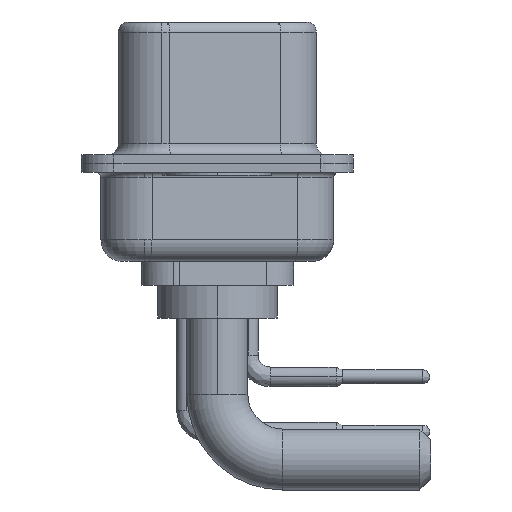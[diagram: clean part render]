
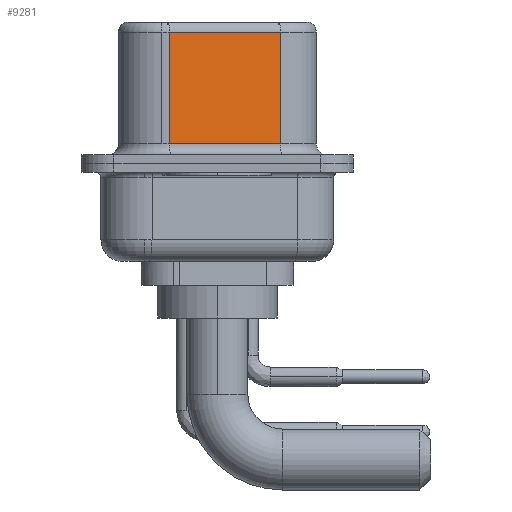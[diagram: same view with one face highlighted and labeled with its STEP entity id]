
A CAD part, left-side view. The second image highlights one B-rep face of the part: STEP entity #9281.
In plain terms, the highlighted planar face has unit normal (-0.985, -0.174, 0).
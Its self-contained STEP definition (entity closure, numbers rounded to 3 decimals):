
#72 = VERTEX_POINT ( 'NONE', #8253 ) ;
#174 = EDGE_LOOP ( 'NONE', ( #11811, #11047, #14633, #18076 ) ) ;
#455 = VECTOR ( 'NONE', #17280, 1000. ) ;
#1044 = AXIS2_PLACEMENT_3D ( 'NONE', #17611, #1335, #7945 ) ;
#1335 = DIRECTION ( 'NONE',  ( 0.985, 0.174, 0. ) ) ;
#3132 = CARTESIAN_POINT ( 'NONE',  ( 4.58, -2.897, 6.02 ) ) ;
#3667 = EDGE_CURVE ( 'NONE', #16047, #14446, #4956, .T. ) ;
#4437 = CARTESIAN_POINT ( 'NONE',  ( 3.68, 2.203, 6.52 ) ) ;
#4581 = CARTESIAN_POINT ( 'NONE',  ( 4.58, -2.897, 6.52 ) ) ;
#4956 = LINE ( 'NONE', #9182, #6905 ) ;
#6149 = DIRECTION ( 'NONE',  ( 0., 0., -1. ) ) ;
#6905 = VECTOR ( 'NONE', #19097, 1000. ) ;
#7233 = EDGE_CURVE ( 'NONE', #72, #16047, #22305, .T. ) ;
#7945 = DIRECTION ( 'NONE',  ( -0.174, 0.985, 0. ) ) ;
#8253 = CARTESIAN_POINT ( 'NONE',  ( 3.68, 2.203, 6.02 ) ) ;
#8675 = CARTESIAN_POINT ( 'NONE',  ( 3.68, 2.203, 0.9 ) ) ;
#9182 = CARTESIAN_POINT ( 'NONE',  ( 4.58, -2.897, 0.9 ) ) ;
#9209 = CARTESIAN_POINT ( 'NONE',  ( 4.58, -2.897, 6.02 ) ) ;
#9281 = ADVANCED_FACE ( 'NONE', ( #13507 ), #22103, .F. ) ;
#10082 = EDGE_CURVE ( 'NONE', #17493, #14446, #25188, .T. ) ;
#11047 = ORIENTED_EDGE ( 'NONE', *, *, #17376, .T. ) ;
#11589 = LINE ( 'NONE', #9209, #455 ) ;
#11811 = ORIENTED_EDGE ( 'NONE', *, *, #10082, .F. ) ;
#12910 = DIRECTION ( 'NONE',  ( 0., 0., -1. ) ) ;
#13507 = FACE_OUTER_BOUND ( 'NONE', #174, .T. ) ;
#14446 = VERTEX_POINT ( 'NONE', #17916 ) ;
#14459 = VECTOR ( 'NONE', #6149, 1000. ) ;
#14633 = ORIENTED_EDGE ( 'NONE', *, *, #7233, .T. ) ;
#16047 = VERTEX_POINT ( 'NONE', #8675 ) ;
#17280 = DIRECTION ( 'NONE',  ( -0.174, 0.985, 0. ) ) ;
#17376 = EDGE_CURVE ( 'NONE', #17493, #72, #11589, .T. ) ;
#17493 = VERTEX_POINT ( 'NONE', #3132 ) ;
#17611 = CARTESIAN_POINT ( 'NONE',  ( 4.58, -2.897, 6.52 ) ) ;
#17916 = CARTESIAN_POINT ( 'NONE',  ( 4.58, -2.897, 0.9 ) ) ;
#18076 = ORIENTED_EDGE ( 'NONE', *, *, #3667, .T. ) ;
#19097 = DIRECTION ( 'NONE',  ( 0.174, -0.985, 0. ) ) ;
#21308 = VECTOR ( 'NONE', #12910, 1000. ) ;
#22103 = PLANE ( 'NONE',  #1044 ) ;
#22305 = LINE ( 'NONE', #4437, #14459 ) ;
#25188 = LINE ( 'NONE', #4581, #21308 ) ;
